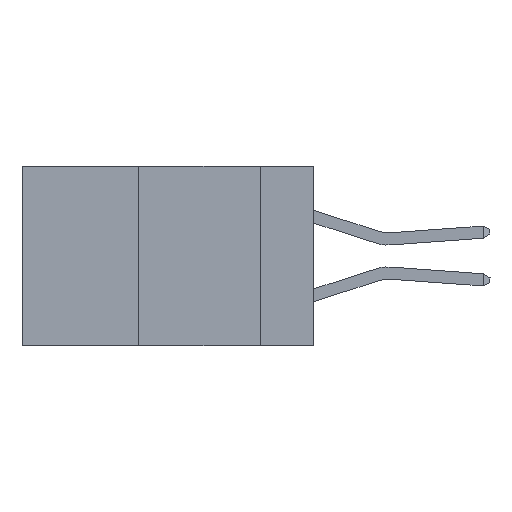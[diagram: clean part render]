
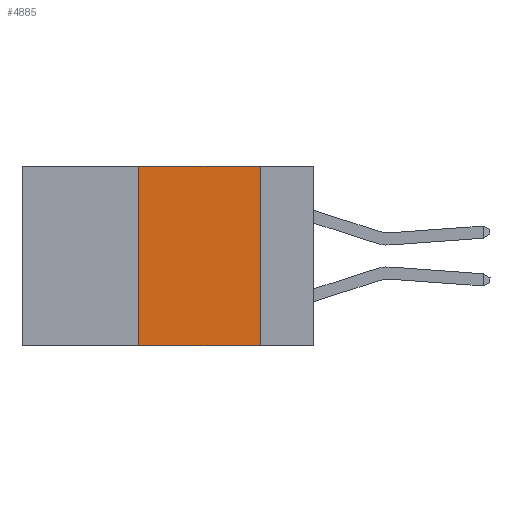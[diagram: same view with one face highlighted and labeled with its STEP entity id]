
A CAD part, left-side view. The second image highlights one B-rep face of the part: STEP entity #4885.
In plain terms, the highlighted planar face has unit normal (-1, 0, 0).
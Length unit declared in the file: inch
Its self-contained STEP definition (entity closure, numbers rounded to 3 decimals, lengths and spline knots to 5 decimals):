
#735 = VECTOR ( 'NONE', #8673, 39.37008 ) ;
#1041 = AXIS2_PLACEMENT_3D ( 'NONE', #14946, #2889, #2376 ) ;
#1258 = ORIENTED_EDGE ( 'NONE', *, *, #2111, .F. ) ;
#1304 = ORIENTED_EDGE ( 'NONE', *, *, #3209, .F. ) ;
#2111 = EDGE_CURVE ( 'NONE', #8195, #3650, #2971, .T. ) ;
#2376 = DIRECTION ( 'NONE',  ( 0., 0., -1. ) ) ;
#2685 = CARTESIAN_POINT ( 'NONE',  ( 0., 0.11, 0. ) ) ;
#2889 = DIRECTION ( 'NONE',  ( 1., 0., 0. ) ) ;
#2971 = LINE ( 'NONE', #16822, #7126 ) ;
#3209 = EDGE_CURVE ( 'NONE', #7872, #8195, #5455, .T. ) ;
#3561 = CARTESIAN_POINT ( 'NONE',  ( 0., 0.11, -0.37 ) ) ;
#3650 = VERTEX_POINT ( 'NONE', #10413 ) ;
#3999 = CARTESIAN_POINT ( 'NONE',  ( 0., 0.36, 0. ) ) ;
#4885 = ADVANCED_FACE ( 'NONE', ( #15856 ), #6379, .F. ) ;
#5455 = LINE ( 'NONE', #14435, #13500 ) ;
#5666 = EDGE_LOOP ( 'NONE', ( #16010, #1258, #1304, #10210 ) ) ;
#5678 = VERTEX_POINT ( 'NONE', #3561 ) ;
#6379 = PLANE ( 'NONE',  #1041 ) ;
#7126 = VECTOR ( 'NONE', #15242, 39.37008 ) ;
#7376 = LINE ( 'NONE', #15670, #18535 ) ;
#7872 = VERTEX_POINT ( 'NONE', #13036 ) ;
#8195 = VERTEX_POINT ( 'NONE', #3999 ) ;
#8394 = DIRECTION ( 'NONE',  ( 0., -1., 0. ) ) ;
#8673 = DIRECTION ( 'NONE',  ( 0., 0., -1. ) ) ;
#10120 = EDGE_CURVE ( 'NONE', #3650, #5678, #12401, .T. ) ;
#10210 = ORIENTED_EDGE ( 'NONE', *, *, #12759, .T. ) ;
#10413 = CARTESIAN_POINT ( 'NONE',  ( 0., 0.11, 0. ) ) ;
#12401 = LINE ( 'NONE', #2685, #735 ) ;
#12759 = EDGE_CURVE ( 'NONE', #7872, #5678, #7376, .T. ) ;
#12928 = DIRECTION ( 'NONE',  ( 0., 0., 1. ) ) ;
#13036 = CARTESIAN_POINT ( 'NONE',  ( 0., 0.36, -0.37 ) ) ;
#13500 = VECTOR ( 'NONE', #12928, 39.37008 ) ;
#14435 = CARTESIAN_POINT ( 'NONE',  ( 0., 0.36, 0. ) ) ;
#14946 = CARTESIAN_POINT ( 'NONE',  ( 0., 0.6, 0. ) ) ;
#15242 = DIRECTION ( 'NONE',  ( 0., -1., 0. ) ) ;
#15670 = CARTESIAN_POINT ( 'NONE',  ( 0., 0.6, -0.37 ) ) ;
#15856 = FACE_OUTER_BOUND ( 'NONE', #5666, .T. ) ;
#16010 = ORIENTED_EDGE ( 'NONE', *, *, #10120, .F. ) ;
#16822 = CARTESIAN_POINT ( 'NONE',  ( 0., 0.6, 0. ) ) ;
#18535 = VECTOR ( 'NONE', #8394, 39.37008 ) ;
